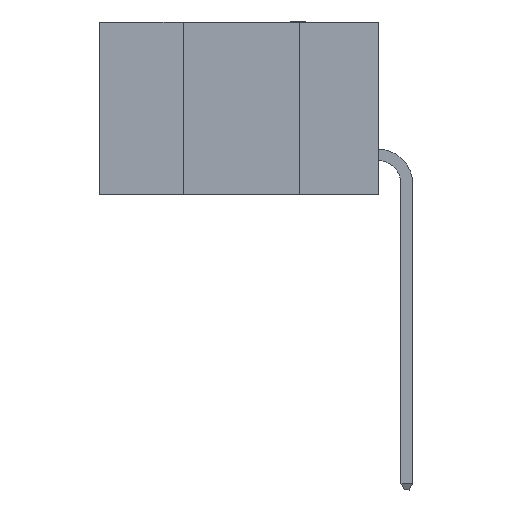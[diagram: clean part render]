
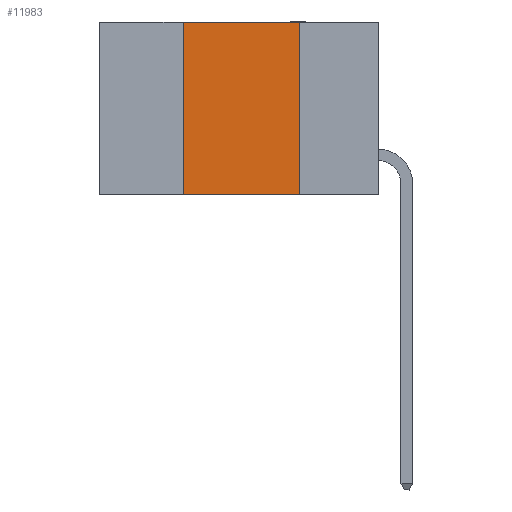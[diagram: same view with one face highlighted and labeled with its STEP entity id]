
A CAD part, left-side view. The second image highlights one B-rep face of the part: STEP entity #11983.
In plain terms, the highlighted planar face has unit normal (-1, 0, 0).
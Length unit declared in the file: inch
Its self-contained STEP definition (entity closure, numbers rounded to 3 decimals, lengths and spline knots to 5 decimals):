
#1288 = EDGE_CURVE ( 'NONE', #15617, #6146, #2797, .T. ) ;
#1905 = VERTEX_POINT ( 'NONE', #8619 ) ;
#2797 = LINE ( 'NONE', #6621, #13719 ) ;
#3225 = EDGE_CURVE ( 'NONE', #1905, #7342, #23623, .T. ) ;
#4984 = CARTESIAN_POINT ( 'NONE',  ( 0., 0.42, 0. ) ) ;
#6146 = VERTEX_POINT ( 'NONE', #4984 ) ;
#6167 = CARTESIAN_POINT ( 'NONE',  ( 0., 0.6, 0. ) ) ;
#6337 = LINE ( 'NONE', #6167, #17064 ) ;
#6621 = CARTESIAN_POINT ( 'NONE',  ( 0., 0.42, 0. ) ) ;
#6906 = ORIENTED_EDGE ( 'NONE', *, *, #18423, .F. ) ;
#7342 = VERTEX_POINT ( 'NONE', #14741 ) ;
#8461 = PLANE ( 'NONE',  #15036 ) ;
#8619 = CARTESIAN_POINT ( 'NONE',  ( 0., 0.17, 0. ) ) ;
#10504 = DIRECTION ( 'NONE',  ( 0., 0., -1. ) ) ;
#11983 = ADVANCED_FACE ( 'NONE', ( #20045 ), #8461, .F. ) ;
#13195 = DIRECTION ( 'NONE',  ( 0., 0., 1. ) ) ;
#13200 = CARTESIAN_POINT ( 'NONE',  ( 0., 0.17, 0. ) ) ;
#13719 = VECTOR ( 'NONE', #13195, 39.37008 ) ;
#13942 = LINE ( 'NONE', #14209, #18499 ) ;
#14189 = DIRECTION ( 'NONE',  ( 0., -1., 0. ) ) ;
#14209 = CARTESIAN_POINT ( 'NONE',  ( 0., 0.6, -0.37 ) ) ;
#14365 = ORIENTED_EDGE ( 'NONE', *, *, #1288, .F. ) ;
#14741 = CARTESIAN_POINT ( 'NONE',  ( 0., 0.17, -0.37 ) ) ;
#15036 = AXIS2_PLACEMENT_3D ( 'NONE', #20389, #22336, #10504 ) ;
#15617 = VERTEX_POINT ( 'NONE', #23292 ) ;
#16194 = DIRECTION ( 'NONE',  ( 0., -1., 0. ) ) ;
#17051 = DIRECTION ( 'NONE',  ( 0., 0., -1. ) ) ;
#17064 = VECTOR ( 'NONE', #14189, 39.37008 ) ;
#18423 = EDGE_CURVE ( 'NONE', #6146, #1905, #6337, .T. ) ;
#18499 = VECTOR ( 'NONE', #16194, 39.37008 ) ;
#18587 = EDGE_LOOP ( 'NONE', ( #23311, #6906, #14365, #20310 ) ) ;
#19380 = EDGE_CURVE ( 'NONE', #15617, #7342, #13942, .T. ) ;
#20045 = FACE_OUTER_BOUND ( 'NONE', #18587, .T. ) ;
#20310 = ORIENTED_EDGE ( 'NONE', *, *, #19380, .T. ) ;
#20389 = CARTESIAN_POINT ( 'NONE',  ( 0., 0.6, 0. ) ) ;
#22336 = DIRECTION ( 'NONE',  ( 1., 0., 0. ) ) ;
#23017 = VECTOR ( 'NONE', #17051, 39.37008 ) ;
#23292 = CARTESIAN_POINT ( 'NONE',  ( 0., 0.42, -0.37 ) ) ;
#23311 = ORIENTED_EDGE ( 'NONE', *, *, #3225, .F. ) ;
#23623 = LINE ( 'NONE', #13200, #23017 ) ;
